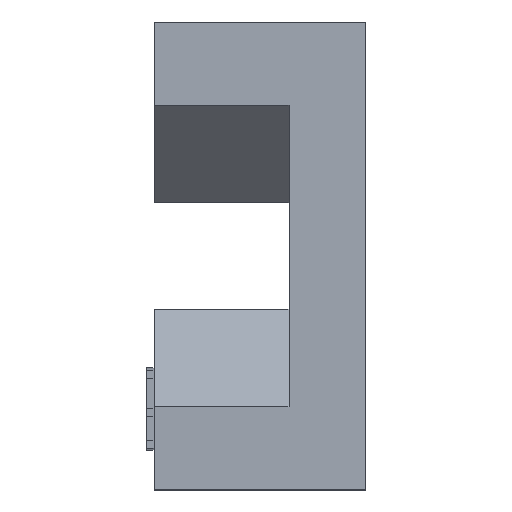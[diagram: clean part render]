
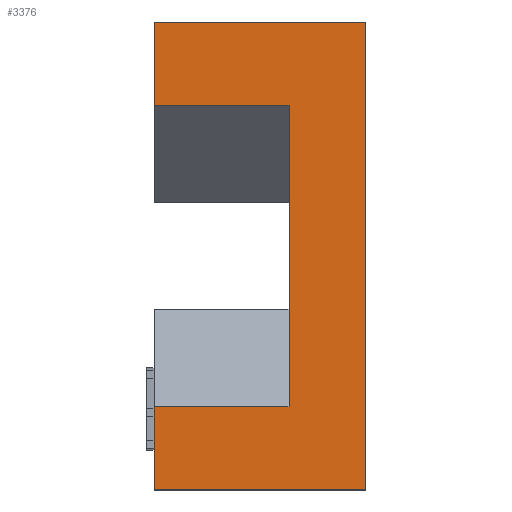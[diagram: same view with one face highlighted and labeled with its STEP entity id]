
A CAD part, left-side view. The second image highlights one B-rep face of the part: STEP entity #3376.
In plain terms, the highlighted planar face has unit normal (-1, 0, 0).
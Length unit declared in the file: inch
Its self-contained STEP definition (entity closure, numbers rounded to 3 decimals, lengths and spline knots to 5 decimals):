
#166 = LINE ( 'NONE', #8513, #13373 ) ;
#188 = EDGE_CURVE ( 'NONE', #9609, #12771, #4861, .T. ) ;
#222 = LINE ( 'NONE', #4500, #9850 ) ;
#530 = EDGE_CURVE ( 'NONE', #7893, #7760, #6923, .T. ) ;
#590 = CARTESIAN_POINT ( 'NONE',  ( -4.5, 0.141, -0.156 ) ) ;
#956 = LINE ( 'NONE', #5290, #3680 ) ;
#1496 = VECTOR ( 'NONE', #11134, 39.37008 ) ;
#1662 = VERTEX_POINT ( 'NONE', #6836 ) ;
#1700 = EDGE_CURVE ( 'NONE', #7760, #9497, #7868, .T. ) ;
#2102 = CARTESIAN_POINT ( 'NONE',  ( -4.5, 0.141, -0.156 ) ) ;
#2637 = ORIENTED_EDGE ( 'NONE', *, *, #9295, .F. ) ;
#2670 = ORIENTED_EDGE ( 'NONE', *, *, #188, .T. ) ;
#3034 = CARTESIAN_POINT ( 'NONE',  ( -4.5, 0.141, 0.156 ) ) ;
#3376 = ADVANCED_FACE ( 'NONE', ( #7341 ), #12453, .F. ) ;
#3489 = EDGE_CURVE ( 'NONE', #9497, #1662, #222, .T. ) ;
#3680 = VECTOR ( 'NONE', #13574, 39.37008 ) ;
#4122 = AXIS2_PLACEMENT_3D ( 'NONE', #2102, #8364, #11356 ) ;
#4196 = DIRECTION ( 'NONE',  ( 0., -1., 0. ) ) ;
#4351 = ORIENTED_EDGE ( 'NONE', *, *, #7652, .T. ) ;
#4500 = CARTESIAN_POINT ( 'NONE',  ( -4.5, 0.141, -0.156 ) ) ;
#4813 = ORIENTED_EDGE ( 'NONE', *, *, #11201, .F. ) ;
#4861 = LINE ( 'NONE', #590, #6780 ) ;
#5190 = CARTESIAN_POINT ( 'NONE',  ( -4.5, 0.141, -0.156 ) ) ;
#5290 = CARTESIAN_POINT ( 'NONE',  ( -4.5, 0.051, -0.1005 ) ) ;
#5705 = CARTESIAN_POINT ( 'NONE',  ( -4.5, 0.141, 0.1005 ) ) ;
#5774 = CARTESIAN_POINT ( 'NONE',  ( -4.5, 0.141, -0.1005 ) ) ;
#5799 = CARTESIAN_POINT ( 'NONE',  ( -4.5, 0.051, 0.1005 ) ) ;
#6157 = CARTESIAN_POINT ( 'NONE',  ( -4.5, 0., -0.156 ) ) ;
#6305 = EDGE_CURVE ( 'NONE', #12771, #9334, #166, .T. ) ;
#6476 = ORIENTED_EDGE ( 'NONE', *, *, #1700, .F. ) ;
#6655 = ORIENTED_EDGE ( 'NONE', *, *, #6305, .T. ) ;
#6780 = VECTOR ( 'NONE', #10110, 39.37008 ) ;
#6836 = CARTESIAN_POINT ( 'NONE',  ( -4.5, 0.141, 0.156 ) ) ;
#6923 = LINE ( 'NONE', #10858, #1496 ) ;
#7341 = FACE_OUTER_BOUND ( 'NONE', #8883, .T. ) ;
#7374 = LINE ( 'NONE', #3034, #13240 ) ;
#7485 = DIRECTION ( 'NONE',  ( 0., 0., 1. ) ) ;
#7637 = CARTESIAN_POINT ( 'NONE',  ( -4.5, 0.051, 0.1005 ) ) ;
#7652 = EDGE_CURVE ( 'NONE', #7893, #9547, #956, .T. ) ;
#7745 = VECTOR ( 'NONE', #8275, 39.37008 ) ;
#7760 = VERTEX_POINT ( 'NONE', #7637 ) ;
#7868 = LINE ( 'NONE', #5799, #9835 ) ;
#7893 = VERTEX_POINT ( 'NONE', #8535 ) ;
#8210 = CARTESIAN_POINT ( 'NONE',  ( -4.5, 0.141, -0.156 ) ) ;
#8275 = DIRECTION ( 'NONE',  ( 0., 0., 1. ) ) ;
#8364 = DIRECTION ( 'NONE',  ( 1., 0., 0. ) ) ;
#8479 = ORIENTED_EDGE ( 'NONE', *, *, #530, .F. ) ;
#8513 = CARTESIAN_POINT ( 'NONE',  ( -4.5, 0., -0.156 ) ) ;
#8535 = CARTESIAN_POINT ( 'NONE',  ( -4.5, 0.051, -0.1005 ) ) ;
#8644 = DIRECTION ( 'NONE',  ( 0., 0., 1. ) ) ;
#8883 = EDGE_LOOP ( 'NONE', ( #8479, #4351, #4813, #2670, #6655, #2637, #13429, #6476 ) ) ;
#9295 = EDGE_CURVE ( 'NONE', #1662, #9334, #7374, .T. ) ;
#9334 = VERTEX_POINT ( 'NONE', #9708 ) ;
#9497 = VERTEX_POINT ( 'NONE', #5705 ) ;
#9547 = VERTEX_POINT ( 'NONE', #5774 ) ;
#9609 = VERTEX_POINT ( 'NONE', #5190 ) ;
#9708 = CARTESIAN_POINT ( 'NONE',  ( -4.5, 0., 0.156 ) ) ;
#9835 = VECTOR ( 'NONE', #11121, 39.37008 ) ;
#9850 = VECTOR ( 'NONE', #8644, 39.37008 ) ;
#10110 = DIRECTION ( 'NONE',  ( 0., -1., 0. ) ) ;
#10858 = CARTESIAN_POINT ( 'NONE',  ( -4.5, 0.051, -0.1005 ) ) ;
#11121 = DIRECTION ( 'NONE',  ( 0., 1., 0. ) ) ;
#11134 = DIRECTION ( 'NONE',  ( 0., 0., 1. ) ) ;
#11201 = EDGE_CURVE ( 'NONE', #9609, #9547, #12574, .T. ) ;
#11356 = DIRECTION ( 'NONE',  ( 0., 0., -1. ) ) ;
#12453 = PLANE ( 'NONE',  #4122 ) ;
#12574 = LINE ( 'NONE', #8210, #7745 ) ;
#12771 = VERTEX_POINT ( 'NONE', #6157 ) ;
#13240 = VECTOR ( 'NONE', #4196, 39.37008 ) ;
#13373 = VECTOR ( 'NONE', #7485, 39.37008 ) ;
#13429 = ORIENTED_EDGE ( 'NONE', *, *, #3489, .F. ) ;
#13574 = DIRECTION ( 'NONE',  ( 0., 1., 0. ) ) ;
